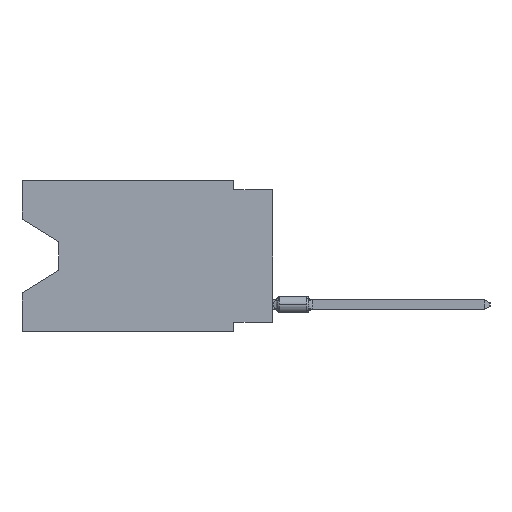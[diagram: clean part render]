
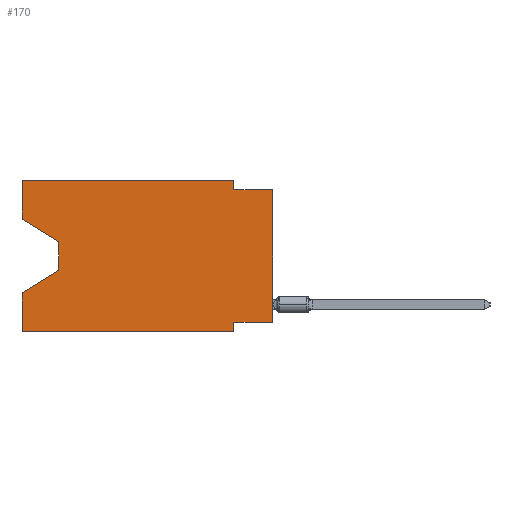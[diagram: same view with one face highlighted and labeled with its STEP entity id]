
A CAD part, left-side view. The second image highlights one B-rep face of the part: STEP entity #170.
In plain terms, the highlighted planar face has unit normal (-1, 0, 0).
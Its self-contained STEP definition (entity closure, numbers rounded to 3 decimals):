
#170 = ADVANCED_FACE ( 'NONE', ( #27641 ), #45981, .F. ) ;
#389 = DIRECTION ( 'NONE',  ( 0., 0., 1. ) ) ;
#442 = EDGE_CURVE ( 'NONE', #46449, #37373, #15958, .T. ) ;
#847 = ORIENTED_EDGE ( 'NONE', *, *, #39749, .T. ) ;
#1041 = CARTESIAN_POINT ( 'NONE',  ( 0., 16.383, -7.36 ) ) ;
#1219 = CARTESIAN_POINT ( 'NONE',  ( 0., 0., -9.271 ) ) ;
#1992 = ORIENTED_EDGE ( 'NONE', *, *, #3697, .F. ) ;
#3697 = EDGE_CURVE ( 'NONE', #43897, #46035, #17745, .T. ) ;
#3725 = LINE ( 'NONE', #43684, #4335 ) ;
#3915 = LINE ( 'NONE', #18397, #45987 ) ;
#4138 = ORIENTED_EDGE ( 'NONE', *, *, #18429, .F. ) ;
#4335 = VECTOR ( 'NONE', #24846, 1000. ) ;
#5353 = LINE ( 'NONE', #16288, #32070 ) ;
#6232 = EDGE_CURVE ( 'NONE', #35670, #14777, #32795, .T. ) ;
#6530 = ORIENTED_EDGE ( 'NONE', *, *, #45648, .F. ) ;
#7419 = VERTEX_POINT ( 'NONE', #23721 ) ;
#9980 = VERTEX_POINT ( 'NONE', #18012 ) ;
#10310 = LINE ( 'NONE', #17442, #27359 ) ;
#10964 = VECTOR ( 'NONE', #22770, 1000. ) ;
#10979 = CARTESIAN_POINT ( 'NONE',  ( 0., 0., -0.635 ) ) ;
#11276 = DIRECTION ( 'NONE',  ( 0., 0., 1. ) ) ;
#12166 = VECTOR ( 'NONE', #389, 1000. ) ;
#12196 = DIRECTION ( 'NONE',  ( 0., 0., -1. ) ) ;
#13502 = EDGE_LOOP ( 'NONE', ( #20189, #18183, #19062, #18729, #847, #24669, #27181, #19400, #23617, #4138, #6530, #1992 ) ) ;
#14158 = VERTEX_POINT ( 'NONE', #31551 ) ;
#14555 = VECTOR ( 'NONE', #26350, 1000. ) ;
#14777 = VERTEX_POINT ( 'NONE', #1041 ) ;
#14829 = DIRECTION ( 'NONE',  ( 0., -1., 0. ) ) ;
#15958 = LINE ( 'NONE', #1219, #46872 ) ;
#16163 = VECTOR ( 'NONE', #12196, 1000. ) ;
#16288 = CARTESIAN_POINT ( 'NONE',  ( 0., 16.383, -2.546 ) ) ;
#16339 = CARTESIAN_POINT ( 'NONE',  ( 0., 2.54, -0.635 ) ) ;
#17442 = CARTESIAN_POINT ( 'NONE',  ( 0., 13.97, -5.893 ) ) ;
#17745 = LINE ( 'NONE', #28690, #12166 ) ;
#18012 = CARTESIAN_POINT ( 'NONE',  ( 0., 13.97, -5.893 ) ) ;
#18183 = ORIENTED_EDGE ( 'NONE', *, *, #37379, .T. ) ;
#18397 = CARTESIAN_POINT ( 'NONE',  ( 0., 16.383, 0. ) ) ;
#18429 = EDGE_CURVE ( 'NONE', #14158, #27927, #27689, .T. ) ;
#18729 = ORIENTED_EDGE ( 'NONE', *, *, #6232, .F. ) ;
#19062 = ORIENTED_EDGE ( 'NONE', *, *, #34212, .T. ) ;
#19400 = ORIENTED_EDGE ( 'NONE', *, *, #31076, .T. ) ;
#19852 = CARTESIAN_POINT ( 'NONE',  ( 0., 0., -0.635 ) ) ;
#19855 = DIRECTION ( 'NONE',  ( 0., 0., -1. ) ) ;
#20189 = ORIENTED_EDGE ( 'NONE', *, *, #41742, .T. ) ;
#20511 = CARTESIAN_POINT ( 'NONE',  ( 0., 16.383, 0. ) ) ;
#22770 = DIRECTION ( 'NONE',  ( 0., -1., 0. ) ) ;
#23346 = CARTESIAN_POINT ( 'NONE',  ( 0., 2.54, -9.271 ) ) ;
#23617 = ORIENTED_EDGE ( 'NONE', *, *, #35623, .F. ) ;
#23721 = CARTESIAN_POINT ( 'NONE',  ( 0., 2.54, -9.906 ) ) ;
#24669 = ORIENTED_EDGE ( 'NONE', *, *, #30536, .F. ) ;
#24846 = DIRECTION ( 'NONE',  ( 0., 0., -1. ) ) ;
#24962 = CARTESIAN_POINT ( 'NONE',  ( 0., 2.54, 0. ) ) ;
#26350 = DIRECTION ( 'NONE',  ( 0., 0., 1. ) ) ;
#27181 = ORIENTED_EDGE ( 'NONE', *, *, #442, .F. ) ;
#27359 = VECTOR ( 'NONE', #31931, 1000. ) ;
#27641 = FACE_OUTER_BOUND ( 'NONE', #13502, .T. ) ;
#27689 = LINE ( 'NONE', #24962, #39947 ) ;
#27927 = VERTEX_POINT ( 'NONE', #16339 ) ;
#28690 = CARTESIAN_POINT ( 'NONE',  ( 0., 16.383, 0. ) ) ;
#29431 = AXIS2_PLACEMENT_3D ( 'NONE', #20511, #31673, #42180 ) ;
#29784 = LINE ( 'NONE', #40762, #43874 ) ;
#30197 = VERTEX_POINT ( 'NONE', #10979 ) ;
#30536 = EDGE_CURVE ( 'NONE', #37373, #7419, #3725, .T. ) ;
#31076 = EDGE_CURVE ( 'NONE', #46449, #30197, #29784, .T. ) ;
#31551 = CARTESIAN_POINT ( 'NONE',  ( 0., 2.54, 0. ) ) ;
#31673 = DIRECTION ( 'NONE',  ( 1., 0., 0. ) ) ;
#31931 = DIRECTION ( 'NONE',  ( 0., 0.855, -0.519 ) ) ;
#32070 = VECTOR ( 'NONE', #45558, 1000. ) ;
#32795 = LINE ( 'NONE', #36829, #14555 ) ;
#33487 = LINE ( 'NONE', #37054, #10964 ) ;
#33823 = CARTESIAN_POINT ( 'NONE',  ( 0., 13.97, -4.013 ) ) ;
#34134 = DIRECTION ( 'NONE',  ( 0., -1., 0. ) ) ;
#34212 = EDGE_CURVE ( 'NONE', #9980, #14777, #10310, .T. ) ;
#34228 = CARTESIAN_POINT ( 'NONE',  ( 0., 16.383, -2.546 ) ) ;
#35426 = DIRECTION ( 'NONE',  ( 0., 1., 0. ) ) ;
#35623 = EDGE_CURVE ( 'NONE', #27927, #30197, #44397, .T. ) ;
#35670 = VERTEX_POINT ( 'NONE', #45342 ) ;
#36153 = CARTESIAN_POINT ( 'NONE',  ( 0., 16.383, 0. ) ) ;
#36829 = CARTESIAN_POINT ( 'NONE',  ( 0., 16.383, 0. ) ) ;
#37054 = CARTESIAN_POINT ( 'NONE',  ( 0., 16.383, -9.906 ) ) ;
#37373 = VERTEX_POINT ( 'NONE', #23346 ) ;
#37379 = EDGE_CURVE ( 'NONE', #44581, #9980, #40522, .T. ) ;
#39689 = CARTESIAN_POINT ( 'NONE',  ( 0., 0., -9.271 ) ) ;
#39749 = EDGE_CURVE ( 'NONE', #35670, #7419, #33487, .T. ) ;
#39947 = VECTOR ( 'NONE', #19855, 1000. ) ;
#40522 = LINE ( 'NONE', #33823, #16163 ) ;
#40762 = CARTESIAN_POINT ( 'NONE',  ( 0., 0., 0. ) ) ;
#41742 = EDGE_CURVE ( 'NONE', #43897, #44581, #5353, .T. ) ;
#42180 = DIRECTION ( 'NONE',  ( 0., 0., -1. ) ) ;
#43684 = CARTESIAN_POINT ( 'NONE',  ( 0., 2.54, -9.906 ) ) ;
#43874 = VECTOR ( 'NONE', #11276, 1000. ) ;
#43897 = VERTEX_POINT ( 'NONE', #34228 ) ;
#44397 = LINE ( 'NONE', #19852, #45695 ) ;
#44581 = VERTEX_POINT ( 'NONE', #44886 ) ;
#44886 = CARTESIAN_POINT ( 'NONE',  ( 0., 13.97, -4.013 ) ) ;
#45342 = CARTESIAN_POINT ( 'NONE',  ( 0., 16.383, -9.906 ) ) ;
#45558 = DIRECTION ( 'NONE',  ( 0., -0.855, -0.519 ) ) ;
#45648 = EDGE_CURVE ( 'NONE', #46035, #14158, #3915, .T. ) ;
#45695 = VECTOR ( 'NONE', #34134, 1000. ) ;
#45981 = PLANE ( 'NONE',  #29431 ) ;
#45987 = VECTOR ( 'NONE', #14829, 1000. ) ;
#46035 = VERTEX_POINT ( 'NONE', #36153 ) ;
#46449 = VERTEX_POINT ( 'NONE', #39689 ) ;
#46872 = VECTOR ( 'NONE', #35426, 1000. ) ;
